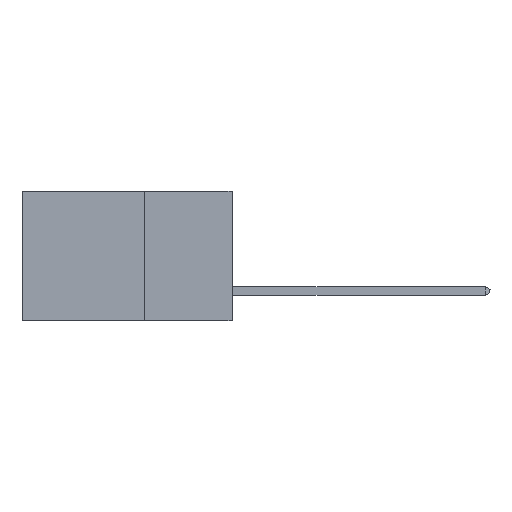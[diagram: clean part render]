
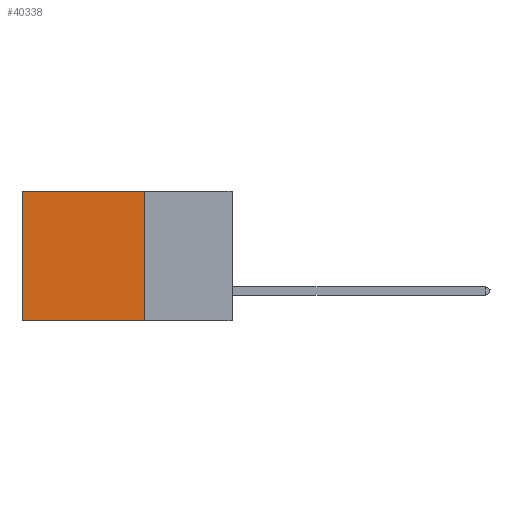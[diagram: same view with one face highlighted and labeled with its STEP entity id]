
A CAD part, left-side view. The second image highlights one B-rep face of the part: STEP entity #40338.
In plain terms, the highlighted planar face has unit normal (-1, 0, 0).
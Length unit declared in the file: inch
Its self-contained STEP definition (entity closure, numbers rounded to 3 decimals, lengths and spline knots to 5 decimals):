
#157 = CARTESIAN_POINT ( 'NONE',  ( 0.2875, 0.6, 0. ) ) ;
#1756 = CARTESIAN_POINT ( 'NONE',  ( 0.2875, 0.25, 0. ) ) ;
#2008 = EDGE_CURVE ( 'NONE', #9566, #23407, #13436, .T. ) ;
#3626 = VECTOR ( 'NONE', #16649, 39.37008 ) ;
#3697 = LINE ( 'NONE', #27669, #30421 ) ;
#6217 = CARTESIAN_POINT ( 'NONE',  ( 0.2875, 0.6, 0. ) ) ;
#6662 = VECTOR ( 'NONE', #25663, 39.37008 ) ;
#7012 = CARTESIAN_POINT ( 'NONE',  ( 0.2875, 0.25, 0. ) ) ;
#7491 = CARTESIAN_POINT ( 'NONE',  ( 0.2875, 0.6, -0.37 ) ) ;
#7702 = ORIENTED_EDGE ( 'NONE', *, *, #23226, .T. ) ;
#9566 = VERTEX_POINT ( 'NONE', #157 ) ;
#10288 = VERTEX_POINT ( 'NONE', #32596 ) ;
#12360 = EDGE_CURVE ( 'NONE', #15301, #10288, #14953, .T. ) ;
#12414 = DIRECTION ( 'NONE',  ( 1., 0., 0. ) ) ;
#13436 = LINE ( 'NONE', #6217, #3626 ) ;
#14953 = LINE ( 'NONE', #22192, #6662 ) ;
#15301 = VERTEX_POINT ( 'NONE', #23199 ) ;
#15951 = DIRECTION ( 'NONE',  ( 0., 0., -1. ) ) ;
#16396 = ORIENTED_EDGE ( 'NONE', *, *, #2008, .T. ) ;
#16649 = DIRECTION ( 'NONE',  ( 0., 0., -1. ) ) ;
#18473 = VECTOR ( 'NONE', #45000, 39.37008 ) ;
#19147 = PLANE ( 'NONE',  #43863 ) ;
#20325 = FACE_OUTER_BOUND ( 'NONE', #25971, .T. ) ;
#20491 = DIRECTION ( 'NONE',  ( 0., 1., 0. ) ) ;
#22192 = CARTESIAN_POINT ( 'NONE',  ( 0.2875, 0.25, 0. ) ) ;
#23199 = CARTESIAN_POINT ( 'NONE',  ( 0.2875, 0.25, 0. ) ) ;
#23226 = EDGE_CURVE ( 'NONE', #15301, #9566, #27155, .T. ) ;
#23407 = VERTEX_POINT ( 'NONE', #7491 ) ;
#25663 = DIRECTION ( 'NONE',  ( 0., 0., -1. ) ) ;
#25971 = EDGE_LOOP ( 'NONE', ( #16396, #37705, #32452, #7702 ) ) ;
#27155 = LINE ( 'NONE', #7012, #18473 ) ;
#27669 = CARTESIAN_POINT ( 'NONE',  ( 0.2875, 0.25, -0.37 ) ) ;
#28145 = EDGE_CURVE ( 'NONE', #10288, #23407, #3697, .T. ) ;
#30421 = VECTOR ( 'NONE', #20491, 39.37008 ) ;
#32452 = ORIENTED_EDGE ( 'NONE', *, *, #12360, .F. ) ;
#32596 = CARTESIAN_POINT ( 'NONE',  ( 0.2875, 0.25, -0.37 ) ) ;
#37705 = ORIENTED_EDGE ( 'NONE', *, *, #28145, .F. ) ;
#40338 = ADVANCED_FACE ( 'NONE', ( #20325 ), #19147, .F. ) ;
#43863 = AXIS2_PLACEMENT_3D ( 'NONE', #1756, #12414, #15951 ) ;
#45000 = DIRECTION ( 'NONE',  ( 0., 1., 0. ) ) ;
